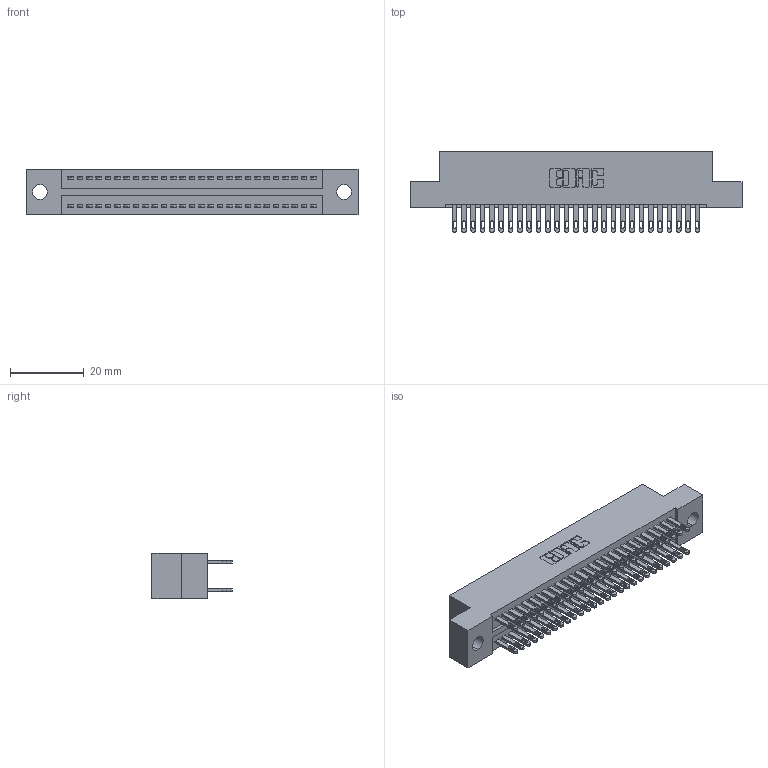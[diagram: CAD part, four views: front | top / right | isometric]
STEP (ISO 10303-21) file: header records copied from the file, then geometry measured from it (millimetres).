
FILE_DESCRIPTION (( 'STEP AP203' ), '1' );
FILE_NAME ('325-054-500-209.STEP', '2020-02-25T00:51:42', ( '' ), ( '' ), 'SwSTEP 2.0', 'SolidWorks 2016', '' );
FILE_SCHEMA (( 'CONFIG_CONTROL_DESIGN' ));
Length unit declared in the file: inch
Products named in the file (3): 325-292-001_325-293-100; 325-054-500-209; 325 Part_.160 TH
Assembly tree (55 placements, depth 2):
  325-054-500-209
    325 Part_.160 TH
    325-292-001_325-293-100  x54
Bounding box: 90.3 x 21.84 x 12.45 mm (x, y, z)
Volume: 11456.6 mm3; surface area: 13996 mm2
Topology: 55 solids, 55 shells, 2706 faces, 8249 edges, 5498 vertices
Faces by surface type: plane 1690, cylinder 1016
Entity records: 19243 total; most frequent: CARTESIAN_POINT 3206, ORIENTED_EDGE 3142, DIRECTION 2767, EDGE_CURVE 1571, LINE 1439, VECTOR 1439, VERTEX_POINT 1046, AXIS2_PLACEMENT_3D 664
